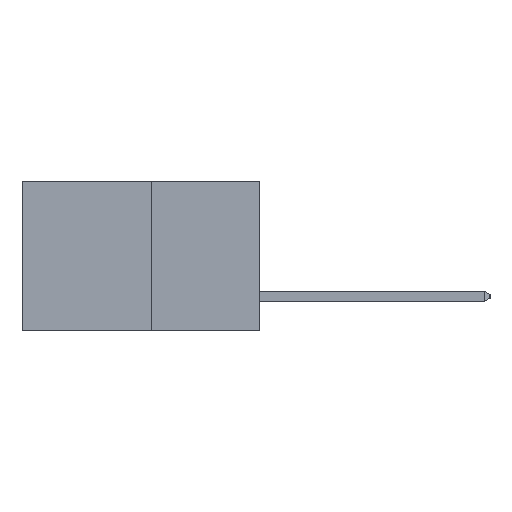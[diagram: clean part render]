
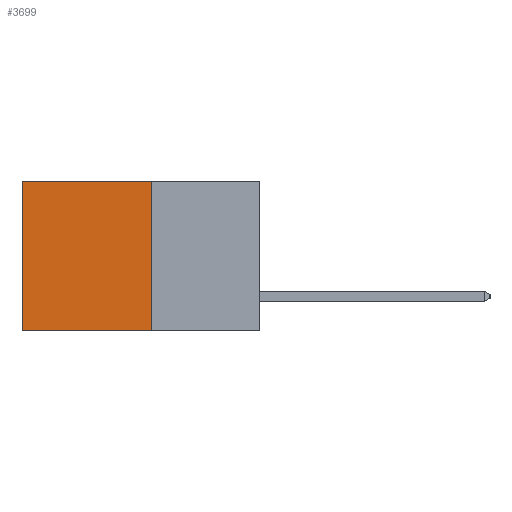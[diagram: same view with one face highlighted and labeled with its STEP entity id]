
A CAD part, left-side view. The second image highlights one B-rep face of the part: STEP entity #3699.
In plain terms, the highlighted planar face has unit normal (-1, 0, 0).
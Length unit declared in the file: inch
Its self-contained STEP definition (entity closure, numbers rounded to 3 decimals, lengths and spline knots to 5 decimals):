
#276 = CARTESIAN_POINT ( 'NONE',  ( 0.277, 0.27, -0.37 ) ) ;
#475 = EDGE_CURVE ( 'NONE', #6291, #1654, #1324, .T. ) ;
#1033 = ORIENTED_EDGE ( 'NONE', *, *, #2804, .T. ) ;
#1061 = CARTESIAN_POINT ( 'NONE',  ( 0.277, 0.59, 0. ) ) ;
#1141 = CARTESIAN_POINT ( 'NONE',  ( 0.277, 0.59, -0.37 ) ) ;
#1324 = LINE ( 'NONE', #9063, #12281 ) ;
#1363 = DIRECTION ( 'NONE',  ( 0., 0., -1. ) ) ;
#1654 = VERTEX_POINT ( 'NONE', #8225 ) ;
#1709 = ORIENTED_EDGE ( 'NONE', *, *, #3789, .T. ) ;
#2177 = VECTOR ( 'NONE', #12556, 39.37008 ) ;
#2804 = EDGE_CURVE ( 'NONE', #11450, #2971, #11008, .T. ) ;
#2971 = VERTEX_POINT ( 'NONE', #1141 ) ;
#3264 = DIRECTION ( 'NONE',  ( 0., 1., 0. ) ) ;
#3699 = ADVANCED_FACE ( 'NONE', ( #13420 ), #4583, .F. ) ;
#3789 = EDGE_CURVE ( 'NONE', #6291, #11450, #6874, .T. ) ;
#4078 = ORIENTED_EDGE ( 'NONE', *, *, #7348, .F. ) ;
#4583 = PLANE ( 'NONE',  #5912 ) ;
#4611 = LINE ( 'NONE', #9634, #12675 ) ;
#5912 = AXIS2_PLACEMENT_3D ( 'NONE', #276, #7812, #1363 ) ;
#6291 = VERTEX_POINT ( 'NONE', #12227 ) ;
#6874 = LINE ( 'NONE', #10002, #9644 ) ;
#7348 = EDGE_CURVE ( 'NONE', #1654, #2971, #4611, .T. ) ;
#7812 = DIRECTION ( 'NONE',  ( 1., 0., 0. ) ) ;
#8225 = CARTESIAN_POINT ( 'NONE',  ( 0.277, 0.27, -0.37 ) ) ;
#9063 = CARTESIAN_POINT ( 'NONE',  ( 0.277, 0.27, -0.37 ) ) ;
#9365 = CARTESIAN_POINT ( 'NONE',  ( 0.277, 0.59, -0.37 ) ) ;
#9506 = EDGE_LOOP ( 'NONE', ( #1033, #4078, #9575, #1709 ) ) ;
#9575 = ORIENTED_EDGE ( 'NONE', *, *, #475, .F. ) ;
#9634 = CARTESIAN_POINT ( 'NONE',  ( 0.277, 0.27, -0.37 ) ) ;
#9644 = VECTOR ( 'NONE', #11085, 39.37008 ) ;
#10002 = CARTESIAN_POINT ( 'NONE',  ( 0.277, 0.27, 0. ) ) ;
#11008 = LINE ( 'NONE', #9365, #2177 ) ;
#11085 = DIRECTION ( 'NONE',  ( 0., 1., 0. ) ) ;
#11450 = VERTEX_POINT ( 'NONE', #1061 ) ;
#11830 = DIRECTION ( 'NONE',  ( 0., 0., -1. ) ) ;
#12227 = CARTESIAN_POINT ( 'NONE',  ( 0.277, 0.27, 0. ) ) ;
#12281 = VECTOR ( 'NONE', #11830, 39.37008 ) ;
#12556 = DIRECTION ( 'NONE',  ( 0., 0., -1. ) ) ;
#12675 = VECTOR ( 'NONE', #3264, 39.37008 ) ;
#13420 = FACE_OUTER_BOUND ( 'NONE', #9506, .T. ) ;
